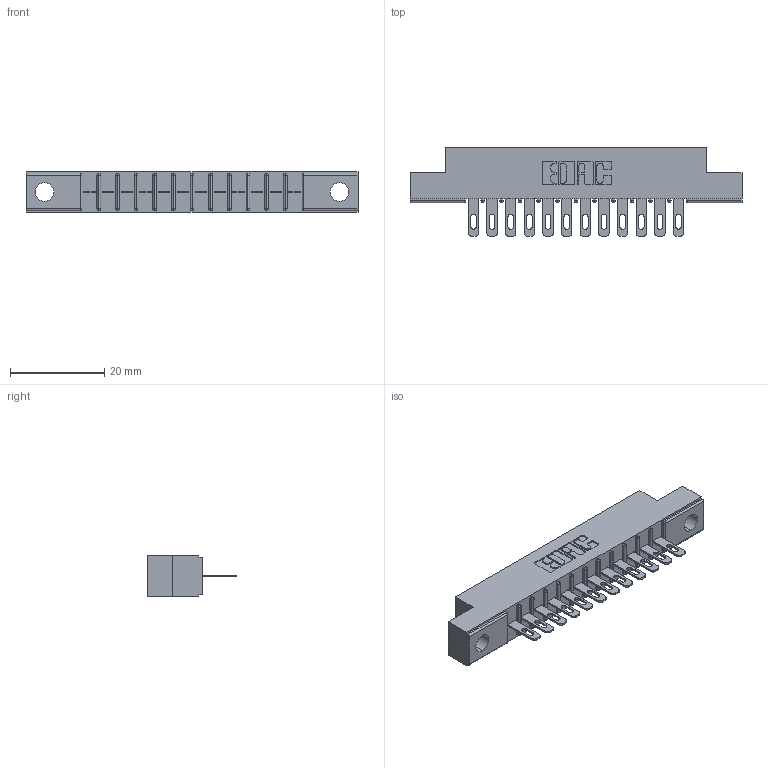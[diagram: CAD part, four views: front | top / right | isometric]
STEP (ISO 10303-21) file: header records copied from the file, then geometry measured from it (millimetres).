
FILE_DESCRIPTION (( 'STEP AP203' ), '1' );
FILE_NAME ('316-012-500-104.STEP', '2018-07-31T00:22:01', ( '' ), ( '' ), 'SwSTEP 2.0', 'SolidWorks 2016', '' );
FILE_SCHEMA (( 'CONFIG_CONTROL_DESIGN' ));
Length unit declared in the file: inch
Products named in the file (3): 306 Part_.156 Dia; 306-290-001_100; 316-012-500-104
Assembly tree (13 placements, depth 2):
  316-012-500-104
    306 Part_.156 Dia
    306-290-001_100  x12
Bounding box: 70.56 x 18.87 x 8.71 mm (x, y, z)
Volume: 4718.3 mm3; surface area: 6705.6 mm2
Topology: 13 solids, 13 shells, 1042 faces, 2932 edges, 1888 vertices
Faces by surface type: plane 682, cylinder 312, sphere 48
Entity records: 15659 total; most frequent: CARTESIAN_POINT 2629, ORIENTED_EDGE 2600, DIRECTION 2588, EDGE_CURVE 1300, LINE 1006, VECTOR 1006, VERTEX_POINT 832, AXIS2_PLACEMENT_3D 791
